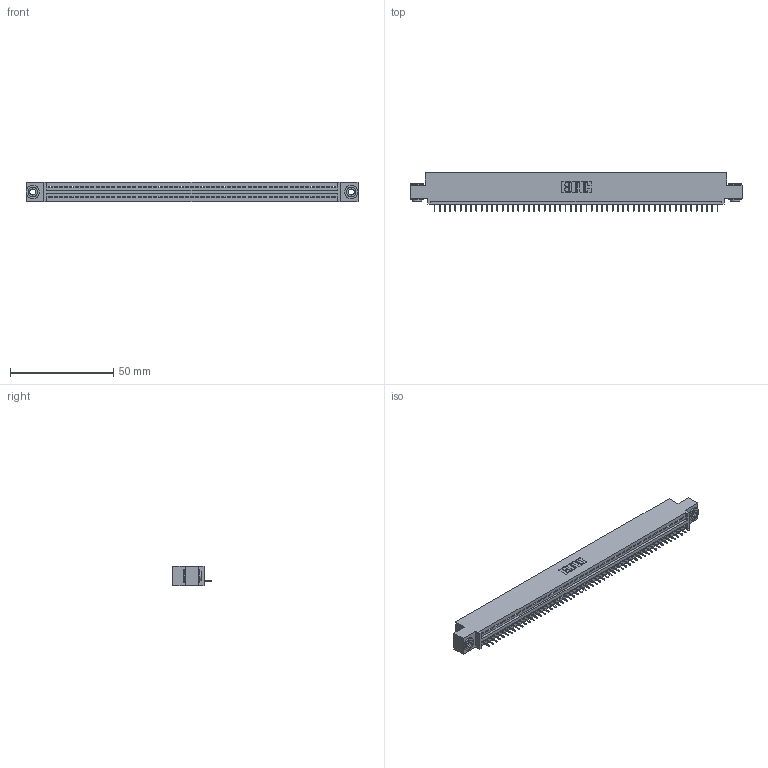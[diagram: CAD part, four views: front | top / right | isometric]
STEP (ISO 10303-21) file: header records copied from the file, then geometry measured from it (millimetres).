
FILE_DESCRIPTION (( 'STEP AP203' ), '1' );
FILE_NAME ('845-055-525-403.STEP', '2020-09-23T12:17:55', ( '' ), ( '' ), 'SwSTEP 2.0', 'SolidWorks 2020', '' );
FILE_SCHEMA (( 'CONFIG_CONTROL_DESIGN' ));
Length unit declared in the file: inch
Products named in the file (4): 345-292-001_345-293-125; 345-250-002_345-250-002-102; 845-055-525-403; 845 Part_0.110 Offset - 0.156 Dia-TH
Assembly tree (58 placements, depth 2):
  845-055-525-403
    845 Part_0.110 Offset - 0.156 Dia-TH
    345-292-001_345-293-125  x55
    345-250-002_345-250-002-102  x2
Bounding box: 160.91 x 18.72 x 9.4 mm (x, y, z)
Volume: 15111.3 mm3; surface area: 19805.7 mm2
Topology: 58 solids, 58 shells, 3578 faces, 10329 edges, 6662 vertices
Faces by surface type: plane 2624, cylinder 946, cone 8
Entity records: 40500 total; most frequent: CARTESIAN_POINT 6992, ORIENTED_EDGE 6974, DIRECTION 6119, EDGE_CURVE 3487, LINE 3115, VECTOR 3115, VERTEX_POINT 2318, AXIS2_PLACEMENT_3D 1502
